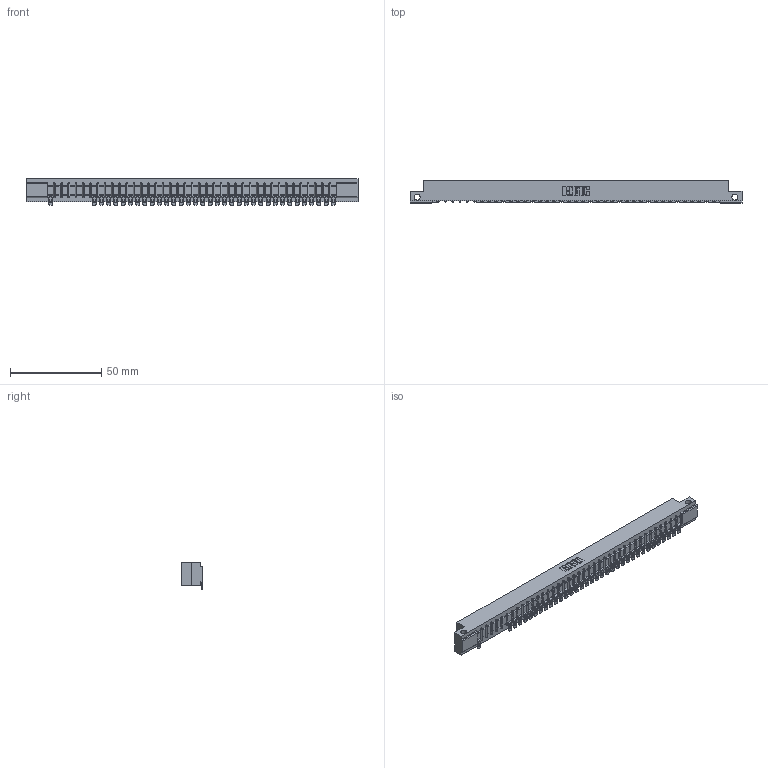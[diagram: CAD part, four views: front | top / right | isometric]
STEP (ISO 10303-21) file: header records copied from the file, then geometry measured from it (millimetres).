
FILE_DESCRIPTION (( 'STEP AP203' ), '1' );
FILE_NAME ('357-040-554-112.STEP', '2018-08-11T05:33:56', ( '' ), ( '' ), 'SwSTEP 2.0', 'SolidWorks 2016', '' );
FILE_SCHEMA (( 'CONFIG_CONTROL_DESIGN' ));
Length unit declared in the file: inch
Products named in the file (3): 307 Part_.128 Dia Side Mounting Holes; 307-290-002_554; 357-040-554-112
Assembly tree (36 placements, depth 2):
  357-040-554-112
    307 Part_.128 Dia Side Mounting Holes
    307-290-002_554  x35
Bounding box: 181.51 x 12.01 x 14.52 mm (x, y, z)
Volume: 19134.6 mm3; surface area: 23212.3 mm2
Topology: 36 solids, 36 shells, 3094 faces, 9498 edges, 6220 vertices
Faces by surface type: plane 1740, cylinder 1272, sphere 82
Entity records: 35345 total; most frequent: CARTESIAN_POINT 5985, ORIENTED_EDGE 5980, DIRECTION 5816, EDGE_CURVE 2990, VECTOR 2282, LINE 2282, VERTEX_POINT 1936, AXIS2_PLACEMENT_3D 1767
